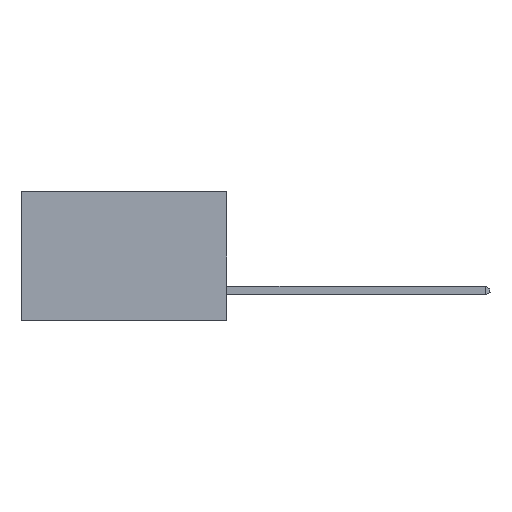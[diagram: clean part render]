
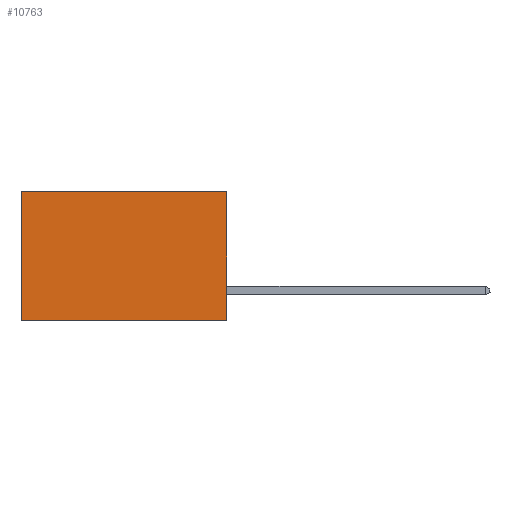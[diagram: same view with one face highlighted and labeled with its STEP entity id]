
A CAD part, left-side view. The second image highlights one B-rep face of the part: STEP entity #10763.
In plain terms, the highlighted planar face has unit normal (-1, 0, 0).
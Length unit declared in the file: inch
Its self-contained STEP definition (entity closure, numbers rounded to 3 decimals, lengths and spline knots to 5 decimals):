
#365 = AXIS2_PLACEMENT_3D ( 'NONE', #18762, #9772, #22346 ) ;
#499 = DIRECTION ( 'NONE',  ( 0., 0., -1. ) ) ;
#1137 = VERTEX_POINT ( 'NONE', #6332 ) ;
#1308 = ORIENTED_EDGE ( 'NONE', *, *, #20323, .T. ) ;
#1540 = DIRECTION ( 'NONE',  ( 0., 0., -1. ) ) ;
#1644 = VECTOR ( 'NONE', #499, 39.37008 ) ;
#1706 = ORIENTED_EDGE ( 'NONE', *, *, #12800, .T. ) ;
#2211 = LINE ( 'NONE', #16515, #1644 ) ;
#2259 = DIRECTION ( 'NONE',  ( 0., 1., 0. ) ) ;
#2407 = LINE ( 'NONE', #21165, #6620 ) ;
#2673 = CARTESIAN_POINT ( 'NONE',  ( 0.277, 0., 0. ) ) ;
#3669 = CARTESIAN_POINT ( 'NONE',  ( 0.277, 0.59, -0.37 ) ) ;
#4445 = VERTEX_POINT ( 'NONE', #3669 ) ;
#4566 = VERTEX_POINT ( 'NONE', #2673 ) ;
#4704 = ORIENTED_EDGE ( 'NONE', *, *, #7780, .F. ) ;
#5589 = EDGE_LOOP ( 'NONE', ( #1706, #4704, #21797, #1308 ) ) ;
#6332 = CARTESIAN_POINT ( 'NONE',  ( 0.277, 0., -0.37 ) ) ;
#6620 = VECTOR ( 'NONE', #1540, 39.37008 ) ;
#7238 = VECTOR ( 'NONE', #2259, 39.37008 ) ;
#7780 = EDGE_CURVE ( 'NONE', #1137, #4445, #8407, .T. ) ;
#8407 = LINE ( 'NONE', #14414, #17415 ) ;
#9772 = DIRECTION ( 'NONE',  ( 1., 0., 0. ) ) ;
#10763 = ADVANCED_FACE ( 'NONE', ( #14851 ), #20570, .F. ) ;
#12476 = LINE ( 'NONE', #12712, #7238 ) ;
#12712 = CARTESIAN_POINT ( 'NONE',  ( 0.277, 0., 0. ) ) ;
#12800 = EDGE_CURVE ( 'NONE', #15965, #4445, #2211, .T. ) ;
#13913 = DIRECTION ( 'NONE',  ( 0., 1., 0. ) ) ;
#14310 = EDGE_CURVE ( 'NONE', #4566, #1137, #2407, .T. ) ;
#14414 = CARTESIAN_POINT ( 'NONE',  ( 0.277, 0., -0.37 ) ) ;
#14851 = FACE_OUTER_BOUND ( 'NONE', #5589, .T. ) ;
#15965 = VERTEX_POINT ( 'NONE', #22196 ) ;
#16515 = CARTESIAN_POINT ( 'NONE',  ( 0.277, 0.59, -0.37 ) ) ;
#17415 = VECTOR ( 'NONE', #13913, 39.37008 ) ;
#18762 = CARTESIAN_POINT ( 'NONE',  ( 0.277, 0., -0.37 ) ) ;
#20323 = EDGE_CURVE ( 'NONE', #4566, #15965, #12476, .T. ) ;
#20570 = PLANE ( 'NONE',  #365 ) ;
#21165 = CARTESIAN_POINT ( 'NONE',  ( 0.277, 0., -0.37 ) ) ;
#21797 = ORIENTED_EDGE ( 'NONE', *, *, #14310, .F. ) ;
#22196 = CARTESIAN_POINT ( 'NONE',  ( 0.277, 0.59, 0. ) ) ;
#22346 = DIRECTION ( 'NONE',  ( 0., 0., -1. ) ) ;
